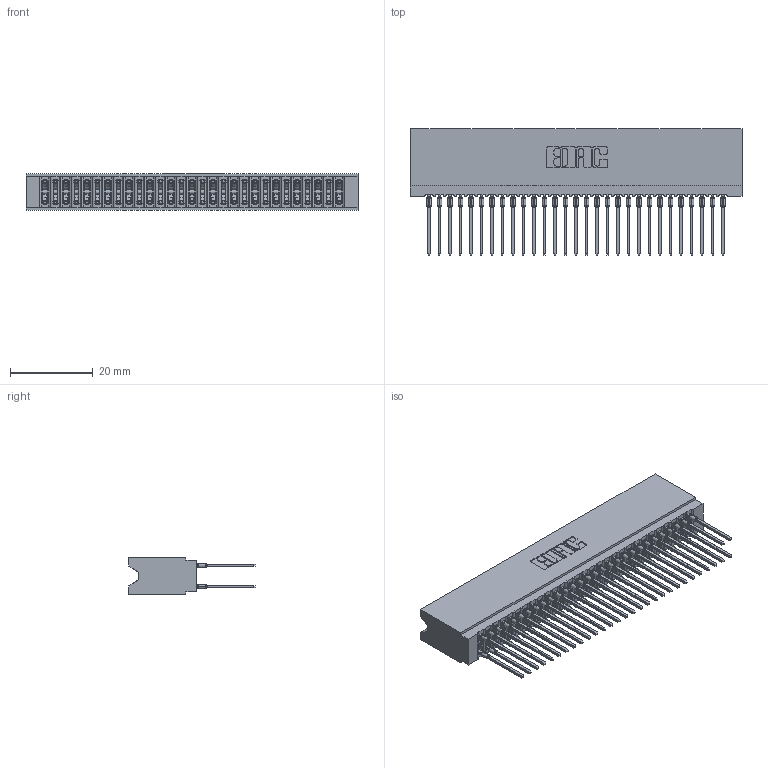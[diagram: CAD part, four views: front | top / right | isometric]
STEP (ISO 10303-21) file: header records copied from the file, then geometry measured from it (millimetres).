
FILE_DESCRIPTION (( 'STEP AP203' ), '1' );
FILE_NAME ('745-058-545-206.STEP', '2026-02-26T18:52:46', ( '' ), ( '' ), 'SwSTEP 2.0', 'SolidWorks 2023', '' );
FILE_SCHEMA (( 'CONFIG_CONTROL_DESIGN' ));
Length unit declared in the file: millimetre
Products named in the file (3): 745 Part_Insulator Option - 06; 745-292-001_545; 745-058-545-206
Assembly tree (59 placements, depth 2):
  745-058-545-206
    745 Part_Insulator Option - 06
    745-292-001_545  x58
Bounding box: 80.26 x 30.62 x 8.89 mm (x, y, z)
Volume: 7488.3 mm3; surface area: 15833.6 mm2
Topology: 59 solids, 59 shells, 5287 faces, 14209 edges, 8930 vertices
Faces by surface type: plane 2724, bspline 1160, cylinder 1055, torus 348
Entity records: 50617 total; most frequent: CARTESIAN_POINT 9286, ORIENTED_EDGE 8696, DIRECTION 7608, EDGE_CURVE 4348, VECTOR 3992, LINE 3992, VERTEX_POINT 2774, AXIS2_PLACEMENT_3D 1808
